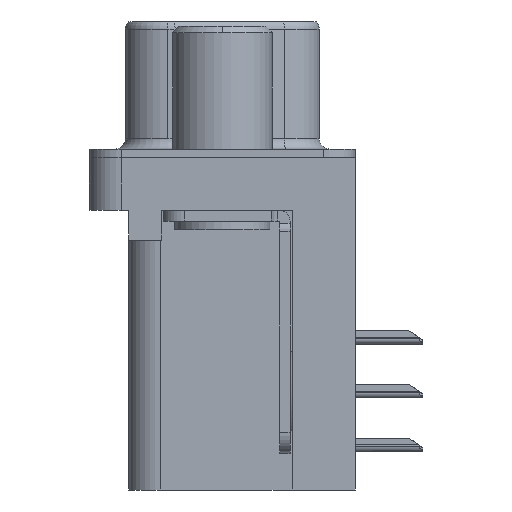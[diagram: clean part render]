
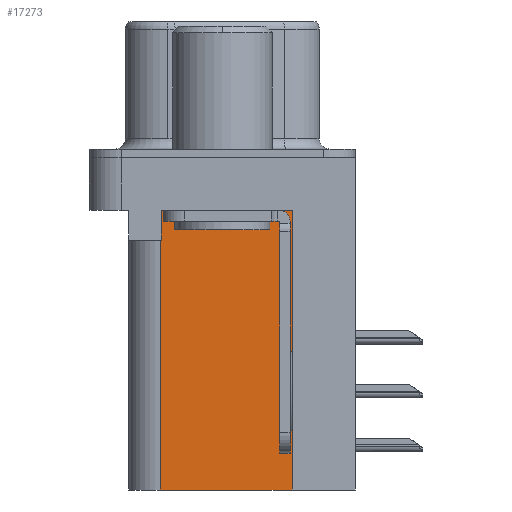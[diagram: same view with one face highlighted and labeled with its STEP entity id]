
A CAD part, left-side view. The second image highlights one B-rep face of the part: STEP entity #17273.
In plain terms, the highlighted planar face has unit normal (-1, 0, 0).
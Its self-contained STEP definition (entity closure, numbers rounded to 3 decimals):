
#1629 = EDGE_CURVE ( 'NONE', #11591, #30079, #7232, .T. ) ;
#1846 = EDGE_CURVE ( 'NONE', #30079, #26055, #5660, .T. ) ;
#2042 = EDGE_CURVE ( 'NONE', #26055, #23082, #4514, .T. ) ;
#4124 = FACE_OUTER_BOUND ( 'NONE', #19061, .T. ) ;
#4482 = VECTOR ( 'NONE', #10038, 1000. ) ;
#4514 = LINE ( 'NONE', #9967, #4482 ) ;
#5582 = ORIENTED_EDGE ( 'NONE', *, *, #13352, .F. ) ;
#5660 = LINE ( 'NONE', #24431, #5778 ) ;
#5778 = VECTOR ( 'NONE', #24519, 1000. ) ;
#6048 = CARTESIAN_POINT ( 'NONE',  ( 3.7, -3.295, -15.7 ) ) ;
#6999 = VECTOR ( 'NONE', #29858, 1000. ) ;
#7232 = LINE ( 'NONE', #25032, #6999 ) ;
#8482 = PLANE ( 'NONE',  #12441 ) ;
#9967 = CARTESIAN_POINT ( 'NONE',  ( 3.7, 0., -3.9 ) ) ;
#10038 = DIRECTION ( 'NONE',  ( 0., 1., 0. ) ) ;
#10977 = DIRECTION ( 'NONE',  ( 0., 0., -1. ) ) ;
#11591 = VERTEX_POINT ( 'NONE', #25388 ) ;
#12441 = AXIS2_PLACEMENT_3D ( 'NONE', #6048, #25287, #10977 ) ;
#13115 = EDGE_CURVE ( 'NONE', #30073, #23082, #21770, .T. ) ;
#13352 = EDGE_CURVE ( 'NONE', #30519, #30073, #20835, .T. ) ;
#13390 = EDGE_CURVE ( 'NONE', #30519, #11591, #20534, .T. ) ;
#14829 = ORIENTED_EDGE ( 'NONE', *, *, #13115, .F. ) ;
#15966 = ORIENTED_EDGE ( 'NONE', *, *, #1629, .T. ) ;
#16254 = CARTESIAN_POINT ( 'NONE',  ( 3.7, -3.295, -15.7 ) ) ;
#17273 = ADVANCED_FACE ( 'NONE', ( #4124 ), #8482, .F. ) ;
#18385 = CARTESIAN_POINT ( 'NONE',  ( 3.7, -3.295, -15.7 ) ) ;
#18590 = CARTESIAN_POINT ( 'NONE',  ( 3.7, 2.895, -2.5 ) ) ;
#18740 = DIRECTION ( 'NONE',  ( 0., 0., 1. ) ) ;
#19061 = EDGE_LOOP ( 'NONE', ( #15966, #21688, #25501, #14829, #5582, #25689 ) ) ;
#19560 = CARTESIAN_POINT ( 'NONE',  ( 3.7, -3.295, -15.7 ) ) ;
#20534 = LINE ( 'NONE', #16254, #20558 ) ;
#20558 = VECTOR ( 'NONE', #30278, 1000. ) ;
#20688 = VECTOR ( 'NONE', #20710, 1000. ) ;
#20710 = DIRECTION ( 'NONE',  ( 0., 1., 0. ) ) ;
#20835 = LINE ( 'NONE', #18385, #20688 ) ;
#21688 = ORIENTED_EDGE ( 'NONE', *, *, #1846, .T. ) ;
#21731 = VECTOR ( 'NONE', #18740, 1000. ) ;
#21770 = LINE ( 'NONE', #28087, #21731 ) ;
#23082 = VERTEX_POINT ( 'NONE', #24125 ) ;
#23348 = CARTESIAN_POINT ( 'NONE',  ( 3.7, 2.925, -15.7 ) ) ;
#24125 = CARTESIAN_POINT ( 'NONE',  ( 3.7, 2.925, -3.9 ) ) ;
#24431 = CARTESIAN_POINT ( 'NONE',  ( 3.7, 2.895, -3.9 ) ) ;
#24519 = DIRECTION ( 'NONE',  ( 0., 0., -1. ) ) ;
#25032 = CARTESIAN_POINT ( 'NONE',  ( 3.7, -3.295, -2.5 ) ) ;
#25287 = DIRECTION ( 'NONE',  ( 1., 0., 0. ) ) ;
#25388 = CARTESIAN_POINT ( 'NONE',  ( 3.7, -3.295, -2.5 ) ) ;
#25501 = ORIENTED_EDGE ( 'NONE', *, *, #2042, .T. ) ;
#25689 = ORIENTED_EDGE ( 'NONE', *, *, #13390, .T. ) ;
#26055 = VERTEX_POINT ( 'NONE', #26139 ) ;
#26139 = CARTESIAN_POINT ( 'NONE',  ( 3.7, 2.895, -3.9 ) ) ;
#28087 = CARTESIAN_POINT ( 'NONE',  ( 3.7, 2.925, -15.7 ) ) ;
#29858 = DIRECTION ( 'NONE',  ( 0., 1., 0. ) ) ;
#30073 = VERTEX_POINT ( 'NONE', #23348 ) ;
#30079 = VERTEX_POINT ( 'NONE', #18590 ) ;
#30278 = DIRECTION ( 'NONE',  ( 0., 0., 1. ) ) ;
#30519 = VERTEX_POINT ( 'NONE', #19560 ) ;
